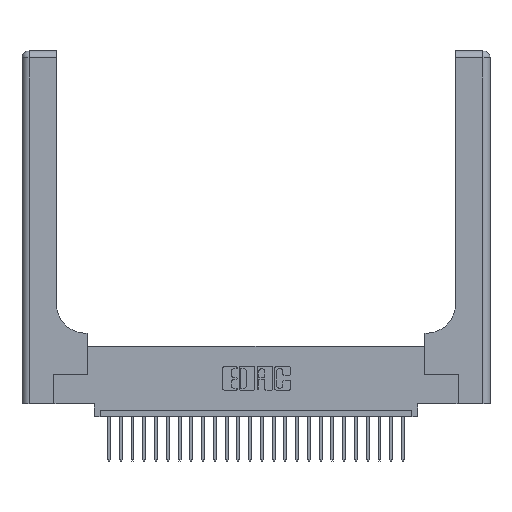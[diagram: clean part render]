
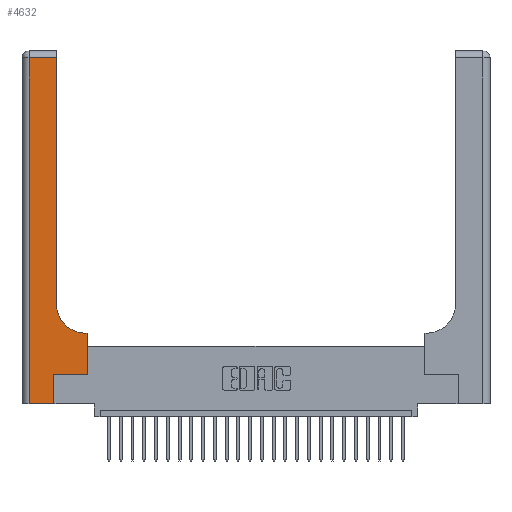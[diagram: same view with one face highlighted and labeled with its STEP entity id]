
A CAD part, top view. The second image highlights one B-rep face of the part: STEP entity #4632.
In plain terms, the highlighted planar face has unit normal (0, 0, 1).
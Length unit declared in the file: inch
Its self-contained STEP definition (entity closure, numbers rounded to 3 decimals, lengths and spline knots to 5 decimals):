
#54 = VECTOR ( 'NONE', #22459, 39.37008 ) ;
#666 = EDGE_CURVE ( 'NONE', #17656, #23670, #12395, .T. ) ;
#1024 = ORIENTED_EDGE ( 'NONE', *, *, #19511, .T. ) ;
#1607 = LINE ( 'NONE', #19945, #6516 ) ;
#2232 = ORIENTED_EDGE ( 'NONE', *, *, #11436, .T. ) ;
#2775 = DIRECTION ( 'NONE',  ( 1., 0., 0. ) ) ;
#2975 = VERTEX_POINT ( 'NONE', #25676 ) ;
#3001 = VECTOR ( 'NONE', #20404, 39.37008 ) ;
#3844 = ORIENTED_EDGE ( 'NONE', *, *, #11469, .T. ) ;
#4208 = EDGE_CURVE ( 'NONE', #2975, #12268, #10923, .T. ) ;
#4221 = CARTESIAN_POINT ( 'NONE',  ( 0.2915, 0.85, 0.37 ) ) ;
#4629 = EDGE_CURVE ( 'NONE', #14658, #7048, #15134, .T. ) ;
#4632 = ADVANCED_FACE ( 'NONE', ( #19676 ), #24638, .F. ) ;
#4726 = VECTOR ( 'NONE', #6494, 39.37008 ) ;
#4827 = EDGE_LOOP ( 'NONE', ( #22688, #26512, #24427, #3844, #19195, #2232, #24552, #1024, #6981 ) ) ;
#6278 = DIRECTION ( 'NONE',  ( -1., 0., 0. ) ) ;
#6494 = DIRECTION ( 'NONE',  ( 1., 0., 0. ) ) ;
#6516 = VECTOR ( 'NONE', #7491, 39.37008 ) ;
#6563 = CARTESIAN_POINT ( 'NONE',  ( 0.2915, 2.94, 0.37 ) ) ;
#6981 = ORIENTED_EDGE ( 'NONE', *, *, #4208, .T. ) ;
#7048 = VERTEX_POINT ( 'NONE', #12829 ) ;
#7491 = DIRECTION ( 'NONE',  ( 0., -1., 0. ) ) ;
#7596 = LINE ( 'NONE', #9888, #3001 ) ;
#7847 = EDGE_CURVE ( 'NONE', #12268, #23739, #7596, .T. ) ;
#7857 = VECTOR ( 'NONE', #16286, 39.37008 ) ;
#8175 = CARTESIAN_POINT ( 'NONE',  ( 0.06, 0., 0.37 ) ) ;
#8279 = CARTESIAN_POINT ( 'NONE',  ( 0., 3., 0.37 ) ) ;
#9128 = DIRECTION ( 'NONE',  ( 0., 1., 0. ) ) ;
#9888 = CARTESIAN_POINT ( 'NONE',  ( 0.2915, 3., 0.37 ) ) ;
#10726 = CARTESIAN_POINT ( 'NONE',  ( 0.269, 0., 0.37 ) ) ;
#10923 = CIRCLE ( 'NONE', #12085, 0.25 ) ;
#11282 = EDGE_CURVE ( 'NONE', #23739, #22876, #14000, .T. ) ;
#11436 = EDGE_CURVE ( 'NONE', #23670, #14658, #14490, .T. ) ;
#11469 = EDGE_CURVE ( 'NONE', #17582, #17656, #18396, .T. ) ;
#11921 = CARTESIAN_POINT ( 'NONE',  ( 0., 2.94, 0.37 ) ) ;
#12085 = AXIS2_PLACEMENT_3D ( 'NONE', #18831, #23008, #2775 ) ;
#12268 = VERTEX_POINT ( 'NONE', #4221 ) ;
#12395 = LINE ( 'NONE', #14106, #7857 ) ;
#12772 = CARTESIAN_POINT ( 'NONE',  ( 0., 0., 0.37 ) ) ;
#12829 = CARTESIAN_POINT ( 'NONE',  ( 0.5585, 0.6, 0.37 ) ) ;
#14000 = LINE ( 'NONE', #11921, #54 ) ;
#14106 = CARTESIAN_POINT ( 'NONE',  ( 0.269, 0., 0.37 ) ) ;
#14490 = LINE ( 'NONE', #16961, #4726 ) ;
#14501 = CARTESIAN_POINT ( 'NONE',  ( 0.5585, 0.25, 0.37 ) ) ;
#14658 = VERTEX_POINT ( 'NONE', #14501 ) ;
#14782 = VECTOR ( 'NONE', #9128, 39.37008 ) ;
#14971 = EDGE_CURVE ( 'NONE', #22876, #17582, #1607, .T. ) ;
#15134 = LINE ( 'NONE', #20225, #14782 ) ;
#16286 = DIRECTION ( 'NONE',  ( 0., 1., 0. ) ) ;
#16510 = DIRECTION ( 'NONE',  ( -1., 0., 0. ) ) ;
#16780 = DIRECTION ( 'NONE',  ( 1., 0., 0. ) ) ;
#16961 = CARTESIAN_POINT ( 'NONE',  ( 0.269, 0.25, 0.37 ) ) ;
#16973 = CARTESIAN_POINT ( 'NONE',  ( 0.06, 2.94, 0.37 ) ) ;
#17100 = VECTOR ( 'NONE', #16780, 39.37008 ) ;
#17582 = VERTEX_POINT ( 'NONE', #8175 ) ;
#17656 = VERTEX_POINT ( 'NONE', #10726 ) ;
#18396 = LINE ( 'NONE', #12772, #17100 ) ;
#18831 = CARTESIAN_POINT ( 'NONE',  ( 0.5415, 0.85, 0.37 ) ) ;
#18879 = VECTOR ( 'NONE', #16510, 39.37008 ) ;
#19195 = ORIENTED_EDGE ( 'NONE', *, *, #666, .T. ) ;
#19511 = EDGE_CURVE ( 'NONE', #7048, #2975, #24403, .T. ) ;
#19676 = FACE_OUTER_BOUND ( 'NONE', #4827, .T. ) ;
#19945 = CARTESIAN_POINT ( 'NONE',  ( 0.06, 3., 0.37 ) ) ;
#20225 = CARTESIAN_POINT ( 'NONE',  ( 0.5585, 0.25, 0.37 ) ) ;
#20404 = DIRECTION ( 'NONE',  ( 0., 1., 0. ) ) ;
#21338 = AXIS2_PLACEMENT_3D ( 'NONE', #8279, #25447, #6278 ) ;
#22459 = DIRECTION ( 'NONE',  ( -1., 0., 0. ) ) ;
#22593 = CARTESIAN_POINT ( 'NONE',  ( 0.2915, 0.6, 0.37 ) ) ;
#22688 = ORIENTED_EDGE ( 'NONE', *, *, #7847, .T. ) ;
#22876 = VERTEX_POINT ( 'NONE', #16973 ) ;
#23008 = DIRECTION ( 'NONE',  ( 0., 0., -1. ) ) ;
#23670 = VERTEX_POINT ( 'NONE', #25203 ) ;
#23739 = VERTEX_POINT ( 'NONE', #6563 ) ;
#24403 = LINE ( 'NONE', #22593, #18879 ) ;
#24427 = ORIENTED_EDGE ( 'NONE', *, *, #14971, .T. ) ;
#24552 = ORIENTED_EDGE ( 'NONE', *, *, #4629, .T. ) ;
#24638 = PLANE ( 'NONE',  #21338 ) ;
#25203 = CARTESIAN_POINT ( 'NONE',  ( 0.269, 0.25, 0.37 ) ) ;
#25447 = DIRECTION ( 'NONE',  ( 0., 0., -1. ) ) ;
#25676 = CARTESIAN_POINT ( 'NONE',  ( 0.5415, 0.6, 0.37 ) ) ;
#26512 = ORIENTED_EDGE ( 'NONE', *, *, #11282, .T. ) ;
